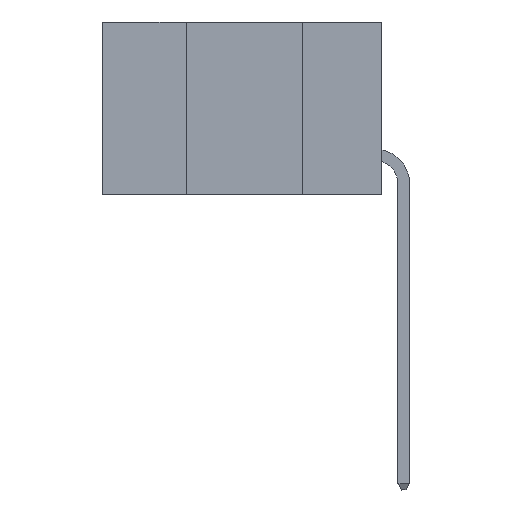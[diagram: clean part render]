
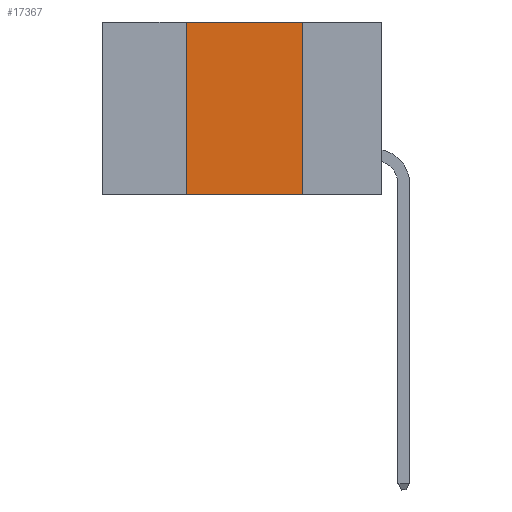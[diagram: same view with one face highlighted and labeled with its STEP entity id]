
A CAD part, left-side view. The second image highlights one B-rep face of the part: STEP entity #17367.
In plain terms, the highlighted planar face has unit normal (-1, 0, 0).
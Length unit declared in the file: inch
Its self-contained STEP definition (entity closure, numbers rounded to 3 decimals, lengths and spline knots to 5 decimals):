
#698 = DIRECTION ( 'NONE',  ( 0., -1., 0. ) ) ;
#972 = DIRECTION ( 'NONE',  ( 1., 0., 0. ) ) ;
#1827 = CARTESIAN_POINT ( 'NONE',  ( 0., 0.6, -0.37 ) ) ;
#2302 = VECTOR ( 'NONE', #10961, 39.37008 ) ;
#2483 = ORIENTED_EDGE ( 'NONE', *, *, #14525, .F. ) ;
#2924 = ORIENTED_EDGE ( 'NONE', *, *, #5488, .F. ) ;
#2987 = CARTESIAN_POINT ( 'NONE',  ( 0., 0.17, 0. ) ) ;
#4536 = DIRECTION ( 'NONE',  ( 0., 0., -1. ) ) ;
#5343 = CARTESIAN_POINT ( 'NONE',  ( 0., 0.17, -0.37 ) ) ;
#5488 = EDGE_CURVE ( 'NONE', #14244, #16147, #16300, .T. ) ;
#6107 = CARTESIAN_POINT ( 'NONE',  ( 0., 0.42, -0.37 ) ) ;
#6624 = EDGE_LOOP ( 'NONE', ( #2483, #10890, #2924, #13821 ) ) ;
#7557 = AXIS2_PLACEMENT_3D ( 'NONE', #15815, #972, #17037 ) ;
#7953 = LINE ( 'NONE', #2987, #12617 ) ;
#9450 = LINE ( 'NONE', #1827, #12621 ) ;
#10752 = CARTESIAN_POINT ( 'NONE',  ( 0., 0.6, 0. ) ) ;
#10890 = ORIENTED_EDGE ( 'NONE', *, *, #14293, .F. ) ;
#10961 = DIRECTION ( 'NONE',  ( 0., 0., 1. ) ) ;
#11142 = CARTESIAN_POINT ( 'NONE',  ( 0., 0.42, 0. ) ) ;
#11641 = CARTESIAN_POINT ( 'NONE',  ( 0., 0.42, 0. ) ) ;
#12617 = VECTOR ( 'NONE', #4536, 39.37008 ) ;
#12621 = VECTOR ( 'NONE', #698, 39.37008 ) ;
#13304 = DIRECTION ( 'NONE',  ( 0., -1., 0. ) ) ;
#13705 = VERTEX_POINT ( 'NONE', #5343 ) ;
#13735 = CARTESIAN_POINT ( 'NONE',  ( 0., 0.17, 0. ) ) ;
#13821 = ORIENTED_EDGE ( 'NONE', *, *, #17181, .T. ) ;
#14244 = VERTEX_POINT ( 'NONE', #6107 ) ;
#14293 = EDGE_CURVE ( 'NONE', #16147, #16625, #16887, .T. ) ;
#14525 = EDGE_CURVE ( 'NONE', #16625, #13705, #7953, .T. ) ;
#15706 = PLANE ( 'NONE',  #7557 ) ;
#15815 = CARTESIAN_POINT ( 'NONE',  ( 0., 0.6, 0. ) ) ;
#16147 = VERTEX_POINT ( 'NONE', #11641 ) ;
#16300 = LINE ( 'NONE', #11142, #2302 ) ;
#16440 = FACE_OUTER_BOUND ( 'NONE', #6624, .T. ) ;
#16449 = VECTOR ( 'NONE', #13304, 39.37008 ) ;
#16625 = VERTEX_POINT ( 'NONE', #13735 ) ;
#16887 = LINE ( 'NONE', #10752, #16449 ) ;
#17037 = DIRECTION ( 'NONE',  ( 0., 0., -1. ) ) ;
#17181 = EDGE_CURVE ( 'NONE', #14244, #13705, #9450, .T. ) ;
#17367 = ADVANCED_FACE ( 'NONE', ( #16440 ), #15706, .F. ) ;
